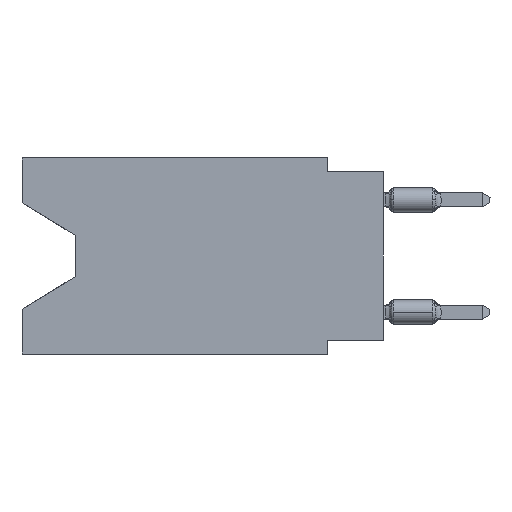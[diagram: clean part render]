
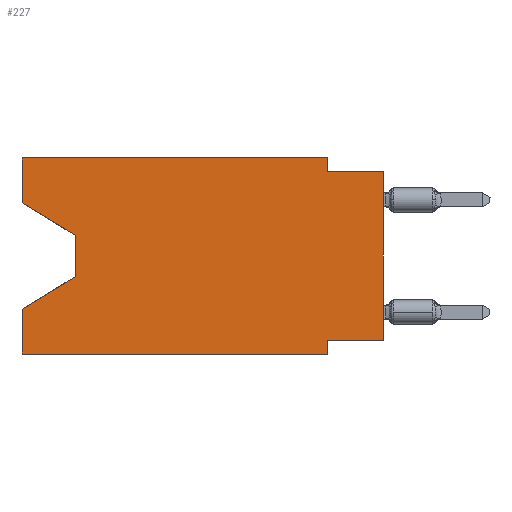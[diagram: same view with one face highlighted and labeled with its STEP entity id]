
A CAD part, left-side view. The second image highlights one B-rep face of the part: STEP entity #227.
In plain terms, the highlighted planar face has unit normal (-1, 0, 0).
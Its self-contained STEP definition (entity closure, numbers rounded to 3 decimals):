
#227 = ADVANCED_FACE ( 'NONE', ( #31464 ), #18550, .F. ) ;
#452 = VECTOR ( 'NONE', #50543, 1000. ) ;
#1193 = VERTEX_POINT ( 'NONE', #28172 ) ;
#1841 = DIRECTION ( 'NONE',  ( 0., 0., 1. ) ) ;
#1949 = LINE ( 'NONE', #33892, #7485 ) ;
#1997 = VECTOR ( 'NONE', #37207, 1000. ) ;
#2259 = VERTEX_POINT ( 'NONE', #8026 ) ;
#2535 = VERTEX_POINT ( 'NONE', #26735 ) ;
#2545 = VERTEX_POINT ( 'NONE', #42819 ) ;
#2973 = DIRECTION ( 'NONE',  ( 1., 0., 0. ) ) ;
#3606 = EDGE_CURVE ( 'NONE', #35496, #18348, #35313, .T. ) ;
#5029 = LINE ( 'NONE', #21639, #1997 ) ;
#5157 = ORIENTED_EDGE ( 'NONE', *, *, #8021, .F. ) ;
#5324 = EDGE_LOOP ( 'NONE', ( #36459, #27161, #12529, #45033, #37419, #16417, #42851, #7989, #40276, #48643, #7124, #5157 ) ) ;
#6177 = LINE ( 'NONE', #26510, #452 ) ;
#6276 = EDGE_CURVE ( 'NONE', #46956, #2535, #10101, .T. ) ;
#7124 = ORIENTED_EDGE ( 'NONE', *, *, #29778, .F. ) ;
#7146 = EDGE_CURVE ( 'NONE', #35496, #34125, #6177, .T. ) ;
#7485 = VECTOR ( 'NONE', #25706, 1000. ) ;
#7989 = ORIENTED_EDGE ( 'NONE', *, *, #7146, .T. ) ;
#8021 = EDGE_CURVE ( 'NONE', #2545, #13982, #21927, .T. ) ;
#8026 = CARTESIAN_POINT ( 'NONE',  ( 0., 16.383, -8.89 ) ) ;
#9030 = AXIS2_PLACEMENT_3D ( 'NONE', #27535, #2973, #22800 ) ;
#9547 = CARTESIAN_POINT ( 'NONE',  ( 0., 16.383, 0. ) ) ;
#10101 = LINE ( 'NONE', #43065, #38253 ) ;
#10305 = EDGE_CURVE ( 'NONE', #41531, #1193, #1949, .T. ) ;
#10451 = VECTOR ( 'NONE', #27579, 1000. ) ;
#11347 = CARTESIAN_POINT ( 'NONE',  ( 0., 16.383, -8.89 ) ) ;
#12529 = ORIENTED_EDGE ( 'NONE', *, *, #6276, .T. ) ;
#12942 = LINE ( 'NONE', #37492, #26540 ) ;
#13177 = VECTOR ( 'NONE', #1841, 1000. ) ;
#13982 = VERTEX_POINT ( 'NONE', #9547 ) ;
#14552 = DIRECTION ( 'NONE',  ( 0., 0.855, -0.519 ) ) ;
#16417 = ORIENTED_EDGE ( 'NONE', *, *, #21321, .F. ) ;
#17247 = VECTOR ( 'NONE', #40335, 1000. ) ;
#17785 = EDGE_CURVE ( 'NONE', #2259, #49632, #47519, .T. ) ;
#18204 = CARTESIAN_POINT ( 'NONE',  ( 0., 16.383, 0. ) ) ;
#18348 = VERTEX_POINT ( 'NONE', #46304 ) ;
#18363 = DIRECTION ( 'NONE',  ( 0., -1., 0. ) ) ;
#18550 = PLANE ( 'NONE',  #9030 ) ;
#19560 = CARTESIAN_POINT ( 'NONE',  ( 0., 16.383, -2.038 ) ) ;
#21000 = CARTESIAN_POINT ( 'NONE',  ( 0., 2.54, -8.89 ) ) ;
#21321 = EDGE_CURVE ( 'NONE', #18348, #49632, #35730, .T. ) ;
#21639 = CARTESIAN_POINT ( 'NONE',  ( 0., 13.97, -3.505 ) ) ;
#21927 = LINE ( 'NONE', #18204, #13177 ) ;
#22800 = DIRECTION ( 'NONE',  ( 0., 0., -1. ) ) ;
#23276 = LINE ( 'NONE', #19560, #38330 ) ;
#23979 = EDGE_CURVE ( 'NONE', #2545, #26449, #23276, .T. ) ;
#24432 = CARTESIAN_POINT ( 'NONE',  ( 0., 13.97, -5.385 ) ) ;
#24592 = CARTESIAN_POINT ( 'NONE',  ( 0., 0., -0.635 ) ) ;
#24596 = DIRECTION ( 'NONE',  ( 0., -1., 0. ) ) ;
#25706 = DIRECTION ( 'NONE',  ( 0., 0., -1. ) ) ;
#26281 = LINE ( 'NONE', #38410, #27692 ) ;
#26449 = VERTEX_POINT ( 'NONE', #27942 ) ;
#26510 = CARTESIAN_POINT ( 'NONE',  ( 0., 0., 0. ) ) ;
#26540 = VECTOR ( 'NONE', #24596, 1000. ) ;
#26735 = CARTESIAN_POINT ( 'NONE',  ( 0., 16.383, -6.852 ) ) ;
#27161 = ORIENTED_EDGE ( 'NONE', *, *, #49191, .T. ) ;
#27217 = DIRECTION ( 'NONE',  ( 0., -0.855, -0.519 ) ) ;
#27475 = DIRECTION ( 'NONE',  ( 0., -1., 0. ) ) ;
#27535 = CARTESIAN_POINT ( 'NONE',  ( 0., 16.383, 0. ) ) ;
#27579 = DIRECTION ( 'NONE',  ( 0., 0., -1. ) ) ;
#27692 = VECTOR ( 'NONE', #18363, 1000. ) ;
#27942 = CARTESIAN_POINT ( 'NONE',  ( 0., 13.97, -3.505 ) ) ;
#28155 = CARTESIAN_POINT ( 'NONE',  ( 0., 2.54, 0. ) ) ;
#28172 = CARTESIAN_POINT ( 'NONE',  ( 0., 2.54, -0.635 ) ) ;
#29778 = EDGE_CURVE ( 'NONE', #13982, #41531, #12942, .T. ) ;
#31088 = DIRECTION ( 'NONE',  ( 0., 1., 0. ) ) ;
#31464 = FACE_OUTER_BOUND ( 'NONE', #5324, .T. ) ;
#32128 = CARTESIAN_POINT ( 'NONE',  ( 0., 0., -8.255 ) ) ;
#32386 = LINE ( 'NONE', #45569, #17247 ) ;
#33892 = CARTESIAN_POINT ( 'NONE',  ( 0., 2.54, 0. ) ) ;
#34125 = VERTEX_POINT ( 'NONE', #24592 ) ;
#35313 = LINE ( 'NONE', #32128, #41253 ) ;
#35496 = VERTEX_POINT ( 'NONE', #41027 ) ;
#35730 = LINE ( 'NONE', #39447, #10451 ) ;
#36459 = ORIENTED_EDGE ( 'NONE', *, *, #23979, .T. ) ;
#37207 = DIRECTION ( 'NONE',  ( 0., 0., -1. ) ) ;
#37419 = ORIENTED_EDGE ( 'NONE', *, *, #17785, .T. ) ;
#37492 = CARTESIAN_POINT ( 'NONE',  ( 0., 16.383, 0. ) ) ;
#38253 = VECTOR ( 'NONE', #14552, 1000. ) ;
#38330 = VECTOR ( 'NONE', #27217, 1000. ) ;
#38410 = CARTESIAN_POINT ( 'NONE',  ( 0., 0., -0.635 ) ) ;
#39447 = CARTESIAN_POINT ( 'NONE',  ( 0., 2.54, -8.89 ) ) ;
#40276 = ORIENTED_EDGE ( 'NONE', *, *, #46681, .F. ) ;
#40335 = DIRECTION ( 'NONE',  ( 0., 0., 1. ) ) ;
#41027 = CARTESIAN_POINT ( 'NONE',  ( 0., 0., -8.255 ) ) ;
#41253 = VECTOR ( 'NONE', #31088, 1000. ) ;
#41531 = VERTEX_POINT ( 'NONE', #28155 ) ;
#42819 = CARTESIAN_POINT ( 'NONE',  ( 0., 16.383, -2.038 ) ) ;
#42851 = ORIENTED_EDGE ( 'NONE', *, *, #3606, .F. ) ;
#43065 = CARTESIAN_POINT ( 'NONE',  ( 0., 13.97, -5.385 ) ) ;
#45033 = ORIENTED_EDGE ( 'NONE', *, *, #47673, .F. ) ;
#45569 = CARTESIAN_POINT ( 'NONE',  ( 0., 16.383, 0. ) ) ;
#45759 = VECTOR ( 'NONE', #27475, 1000. ) ;
#46304 = CARTESIAN_POINT ( 'NONE',  ( 0., 2.54, -8.255 ) ) ;
#46681 = EDGE_CURVE ( 'NONE', #1193, #34125, #26281, .T. ) ;
#46956 = VERTEX_POINT ( 'NONE', #24432 ) ;
#47519 = LINE ( 'NONE', #11347, #45759 ) ;
#47673 = EDGE_CURVE ( 'NONE', #2259, #2535, #32386, .T. ) ;
#48643 = ORIENTED_EDGE ( 'NONE', *, *, #10305, .F. ) ;
#49191 = EDGE_CURVE ( 'NONE', #26449, #46956, #5029, .T. ) ;
#49632 = VERTEX_POINT ( 'NONE', #21000 ) ;
#50543 = DIRECTION ( 'NONE',  ( 0., 0., 1. ) ) ;
